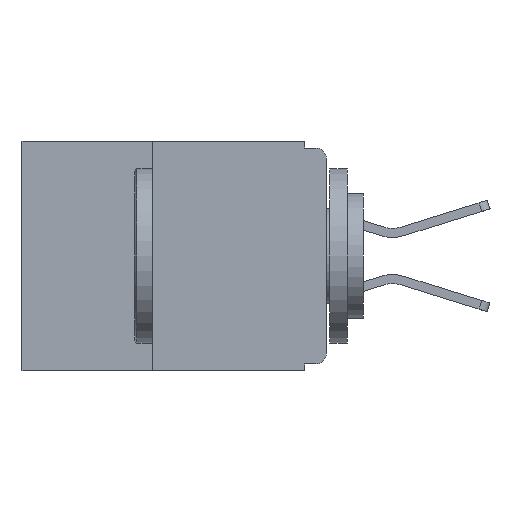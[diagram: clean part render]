
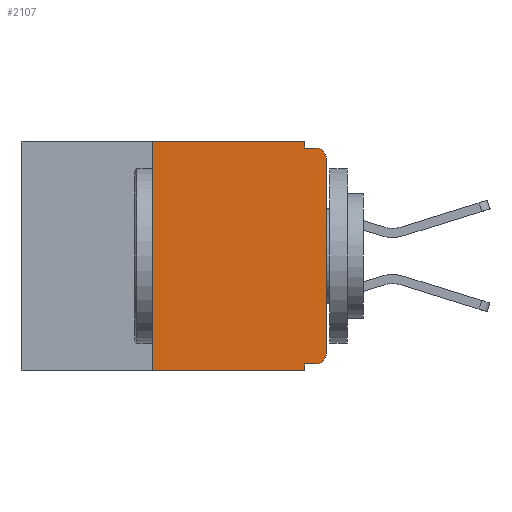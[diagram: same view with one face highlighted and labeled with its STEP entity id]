
A CAD part, left-side view. The second image highlights one B-rep face of the part: STEP entity #2107.
In plain terms, the highlighted planar face has unit normal (-1, 0, 0).
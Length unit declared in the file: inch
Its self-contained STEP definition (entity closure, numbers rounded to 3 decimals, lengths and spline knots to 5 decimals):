
#264 = EDGE_CURVE ( 'NONE', #12044, #5505, #10988, .T. ) ;
#507 = VECTOR ( 'NONE', #512, 39.37008 ) ;
#512 = DIRECTION ( 'NONE',  ( 0., -1., 0. ) ) ;
#814 = VECTOR ( 'NONE', #13849, 39.37008 ) ;
#1671 = ORIENTED_EDGE ( 'NONE', *, *, #4063, .F. ) ;
#1973 = VECTOR ( 'NONE', #2913, 39.37008 ) ;
#2103 = CARTESIAN_POINT ( 'NONE',  ( 0., 0.015, -0.025 ) ) ;
#2107 = ADVANCED_FACE ( 'NONE', ( #14251 ), #3410, .F. ) ;
#2139 = LINE ( 'NONE', #3212, #10752 ) ;
#2913 = DIRECTION ( 'NONE',  ( 0., 0., -1. ) ) ;
#2935 = ORIENTED_EDGE ( 'NONE', *, *, #4398, .T. ) ;
#3212 = CARTESIAN_POINT ( 'NONE',  ( 0., 0., -0.32 ) ) ;
#3275 = DIRECTION ( 'NONE',  ( 0., 0., -1. ) ) ;
#3367 = DIRECTION ( 'NONE',  ( 0., 0., 1. ) ) ;
#3410 = PLANE ( 'NONE',  #13638 ) ;
#3534 = CARTESIAN_POINT ( 'NONE',  ( 0., 0.031, -0.01 ) ) ;
#3612 = VERTEX_POINT ( 'NONE', #6391 ) ;
#3709 = CARTESIAN_POINT ( 'NONE',  ( 0., 0.015, -0.01 ) ) ;
#3775 = DIRECTION ( 'NONE',  ( 0., 0., 1. ) ) ;
#3902 = LINE ( 'NONE', #6311, #814 ) ;
#4046 = ORIENTED_EDGE ( 'NONE', *, *, #12706, .F. ) ;
#4063 = EDGE_CURVE ( 'NONE', #12044, #12688, #2139, .T. ) ;
#4341 = ORIENTED_EDGE ( 'NONE', *, *, #10812, .T. ) ;
#4398 = EDGE_CURVE ( 'NONE', #8562, #9064, #9552, .T. ) ;
#4493 = CARTESIAN_POINT ( 'NONE',  ( 0., 0.015, -0.305 ) ) ;
#4702 = EDGE_LOOP ( 'NONE', ( #4341, #11402, #9563, #5087, #5317, #5098, #2935, #4046, #1671, #6366 ) ) ;
#4848 = DIRECTION ( 'NONE',  ( 0., -1., 0. ) ) ;
#5067 = LINE ( 'NONE', #7396, #1973 ) ;
#5087 = ORIENTED_EDGE ( 'NONE', *, *, #12454, .F. ) ;
#5098 = ORIENTED_EDGE ( 'NONE', *, *, #11050, .F. ) ;
#5317 = ORIENTED_EDGE ( 'NONE', *, *, #12250, .F. ) ;
#5505 = VERTEX_POINT ( 'NONE', #9269 ) ;
#5839 = VECTOR ( 'NONE', #3775, 39.37008 ) ;
#6311 = CARTESIAN_POINT ( 'NONE',  ( 0., 0., -0.01 ) ) ;
#6331 = CARTESIAN_POINT ( 'NONE',  ( 0., 0.031, -0.33 ) ) ;
#6366 = ORIENTED_EDGE ( 'NONE', *, *, #264, .T. ) ;
#6391 = CARTESIAN_POINT ( 'NONE',  ( 0., 0.031, 0. ) ) ;
#6585 = AXIS2_PLACEMENT_3D ( 'NONE', #4493, #10760, #12629 ) ;
#6817 = CARTESIAN_POINT ( 'NONE',  ( 0., 0.25, 0. ) ) ;
#6831 = LINE ( 'NONE', #12476, #12590 ) ;
#7063 = DIRECTION ( 'NONE',  ( 0., 0., -1. ) ) ;
#7311 = CARTESIAN_POINT ( 'NONE',  ( 0., 0.031, -0.32 ) ) ;
#7396 = CARTESIAN_POINT ( 'NONE',  ( 0., 0.031, 0. ) ) ;
#7490 = DIRECTION ( 'NONE',  ( 1., 0., 0. ) ) ;
#7526 = VERTEX_POINT ( 'NONE', #3709 ) ;
#7685 = CARTESIAN_POINT ( 'NONE',  ( 0., 0.437, 0. ) ) ;
#7691 = VERTEX_POINT ( 'NONE', #11707 ) ;
#8034 = AXIS2_PLACEMENT_3D ( 'NONE', #2103, #10014, #3275 ) ;
#8095 = VERTEX_POINT ( 'NONE', #3534 ) ;
#8249 = CARTESIAN_POINT ( 'NONE',  ( 0., 0.25, -0.33 ) ) ;
#8518 = CARTESIAN_POINT ( 'NONE',  ( 0., 0.031, -0.33 ) ) ;
#8562 = VERTEX_POINT ( 'NONE', #8760 ) ;
#8760 = CARTESIAN_POINT ( 'NONE',  ( 0., 0.25, -0.33 ) ) ;
#8813 = LINE ( 'NONE', #8249, #5839 ) ;
#8983 = VECTOR ( 'NONE', #3367, 39.37008 ) ;
#9064 = VERTEX_POINT ( 'NONE', #6331 ) ;
#9269 = CARTESIAN_POINT ( 'NONE',  ( 0., 0., -0.305 ) ) ;
#9552 = LINE ( 'NONE', #13782, #507 ) ;
#9560 = DIRECTION ( 'NONE',  ( 0., 0., -1. ) ) ;
#9563 = ORIENTED_EDGE ( 'NONE', *, *, #10577, .F. ) ;
#9704 = VERTEX_POINT ( 'NONE', #6817 ) ;
#9951 = DIRECTION ( 'NONE',  ( 0., 1., 0. ) ) ;
#10014 = DIRECTION ( 'NONE',  ( -1., 0., 0. ) ) ;
#10099 = CARTESIAN_POINT ( 'NONE',  ( 0., 0., 0. ) ) ;
#10127 = CIRCLE ( 'NONE', #8034, 0.015 ) ;
#10302 = LINE ( 'NONE', #8518, #13071 ) ;
#10577 = EDGE_CURVE ( 'NONE', #8095, #7526, #3902, .T. ) ;
#10752 = VECTOR ( 'NONE', #9951, 39.37008 ) ;
#10760 = DIRECTION ( 'NONE',  ( -1., 0., 0. ) ) ;
#10812 = EDGE_CURVE ( 'NONE', #5505, #7691, #11825, .T. ) ;
#10988 = CIRCLE ( 'NONE', #6585, 0.015 ) ;
#11050 = EDGE_CURVE ( 'NONE', #8562, #9704, #8813, .T. ) ;
#11402 = ORIENTED_EDGE ( 'NONE', *, *, #12930, .T. ) ;
#11707 = CARTESIAN_POINT ( 'NONE',  ( 0., 0., -0.025 ) ) ;
#11825 = LINE ( 'NONE', #10099, #8983 ) ;
#12044 = VERTEX_POINT ( 'NONE', #12115 ) ;
#12115 = CARTESIAN_POINT ( 'NONE',  ( 0., 0.015, -0.32 ) ) ;
#12250 = EDGE_CURVE ( 'NONE', #9704, #3612, #6831, .T. ) ;
#12454 = EDGE_CURVE ( 'NONE', #3612, #8095, #5067, .T. ) ;
#12476 = CARTESIAN_POINT ( 'NONE',  ( 0., 0.437, 0. ) ) ;
#12590 = VECTOR ( 'NONE', #4848, 39.37008 ) ;
#12629 = DIRECTION ( 'NONE',  ( 0., 0., -1. ) ) ;
#12688 = VERTEX_POINT ( 'NONE', #7311 ) ;
#12706 = EDGE_CURVE ( 'NONE', #12688, #9064, #10302, .T. ) ;
#12930 = EDGE_CURVE ( 'NONE', #7691, #7526, #10127, .T. ) ;
#13071 = VECTOR ( 'NONE', #9560, 39.37008 ) ;
#13638 = AXIS2_PLACEMENT_3D ( 'NONE', #7685, #7490, #7063 ) ;
#13782 = CARTESIAN_POINT ( 'NONE',  ( 0., 0.437, -0.33 ) ) ;
#13849 = DIRECTION ( 'NONE',  ( 0., -1., 0. ) ) ;
#14251 = FACE_OUTER_BOUND ( 'NONE', #4702, .T. ) ;
